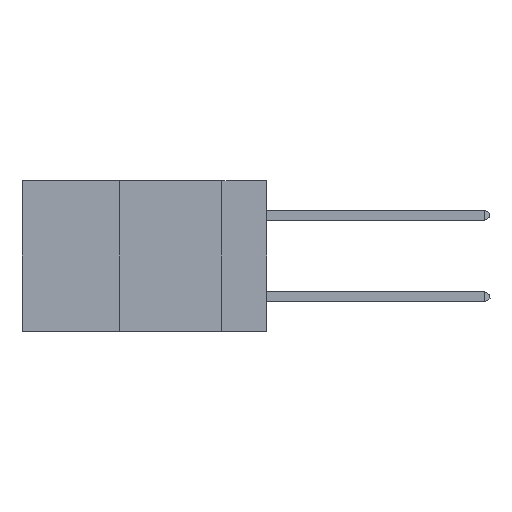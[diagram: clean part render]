
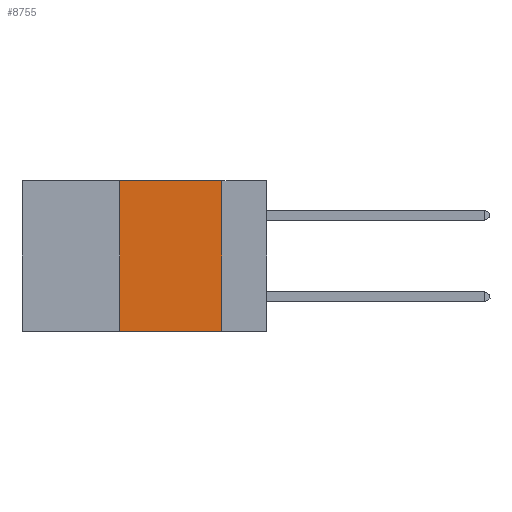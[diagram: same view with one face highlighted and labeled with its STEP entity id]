
A CAD part, left-side view. The second image highlights one B-rep face of the part: STEP entity #8755.
In plain terms, the highlighted planar face has unit normal (-1, 0, 0).
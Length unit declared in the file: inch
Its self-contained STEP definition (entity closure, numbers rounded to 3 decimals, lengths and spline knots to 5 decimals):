
#572 = ORIENTED_EDGE ( 'NONE', *, *, #2477, .F. ) ;
#667 = EDGE_LOOP ( 'NONE', ( #3080, #12222, #572, #10953 ) ) ;
#682 = DIRECTION ( 'NONE',  ( 0., -1., 0. ) ) ;
#1345 = AXIS2_PLACEMENT_3D ( 'NONE', #4629, #9263, #10196 ) ;
#1378 = VERTEX_POINT ( 'NONE', #12190 ) ;
#2017 = VECTOR ( 'NONE', #682, 39.37008 ) ;
#2477 = EDGE_CURVE ( 'NONE', #3710, #1378, #4456, .T. ) ;
#2592 = PLANE ( 'NONE',  #1345 ) ;
#2699 = LINE ( 'NONE', #4859, #7177 ) ;
#2924 = EDGE_CURVE ( 'NONE', #6778, #11511, #5053, .T. ) ;
#2959 = CARTESIAN_POINT ( 'NONE',  ( 0., 0.36, -0.37 ) ) ;
#3080 = ORIENTED_EDGE ( 'NONE', *, *, #2924, .F. ) ;
#3357 = LINE ( 'NONE', #6557, #2017 ) ;
#3710 = VERTEX_POINT ( 'NONE', #2959 ) ;
#4456 = LINE ( 'NONE', #5076, #11162 ) ;
#4629 = CARTESIAN_POINT ( 'NONE',  ( 0., 0.6, 0. ) ) ;
#4859 = CARTESIAN_POINT ( 'NONE',  ( 0., 0.6, -0.37 ) ) ;
#4907 = VECTOR ( 'NONE', #7576, 39.37008 ) ;
#5053 = LINE ( 'NONE', #10422, #4907 ) ;
#5076 = CARTESIAN_POINT ( 'NONE',  ( 0., 0.36, 0. ) ) ;
#6557 = CARTESIAN_POINT ( 'NONE',  ( 0., 0.6, 0. ) ) ;
#6778 = VERTEX_POINT ( 'NONE', #11854 ) ;
#7177 = VECTOR ( 'NONE', #11893, 39.37008 ) ;
#7576 = DIRECTION ( 'NONE',  ( 0., 0., -1. ) ) ;
#8755 = ADVANCED_FACE ( 'NONE', ( #9623 ), #2592, .F. ) ;
#8802 = EDGE_CURVE ( 'NONE', #1378, #6778, #3357, .T. ) ;
#9263 = DIRECTION ( 'NONE',  ( 1., 0., 0. ) ) ;
#9623 = FACE_OUTER_BOUND ( 'NONE', #667, .T. ) ;
#9734 = DIRECTION ( 'NONE',  ( 0., 0., 1. ) ) ;
#10196 = DIRECTION ( 'NONE',  ( 0., 0., -1. ) ) ;
#10422 = CARTESIAN_POINT ( 'NONE',  ( 0., 0.11, 0. ) ) ;
#10953 = ORIENTED_EDGE ( 'NONE', *, *, #11945, .T. ) ;
#11162 = VECTOR ( 'NONE', #9734, 39.37008 ) ;
#11511 = VERTEX_POINT ( 'NONE', #12069 ) ;
#11854 = CARTESIAN_POINT ( 'NONE',  ( 0., 0.11, 0. ) ) ;
#11893 = DIRECTION ( 'NONE',  ( 0., -1., 0. ) ) ;
#11945 = EDGE_CURVE ( 'NONE', #3710, #11511, #2699, .T. ) ;
#12069 = CARTESIAN_POINT ( 'NONE',  ( 0., 0.11, -0.37 ) ) ;
#12190 = CARTESIAN_POINT ( 'NONE',  ( 0., 0.36, 0. ) ) ;
#12222 = ORIENTED_EDGE ( 'NONE', *, *, #8802, .F. ) ;
